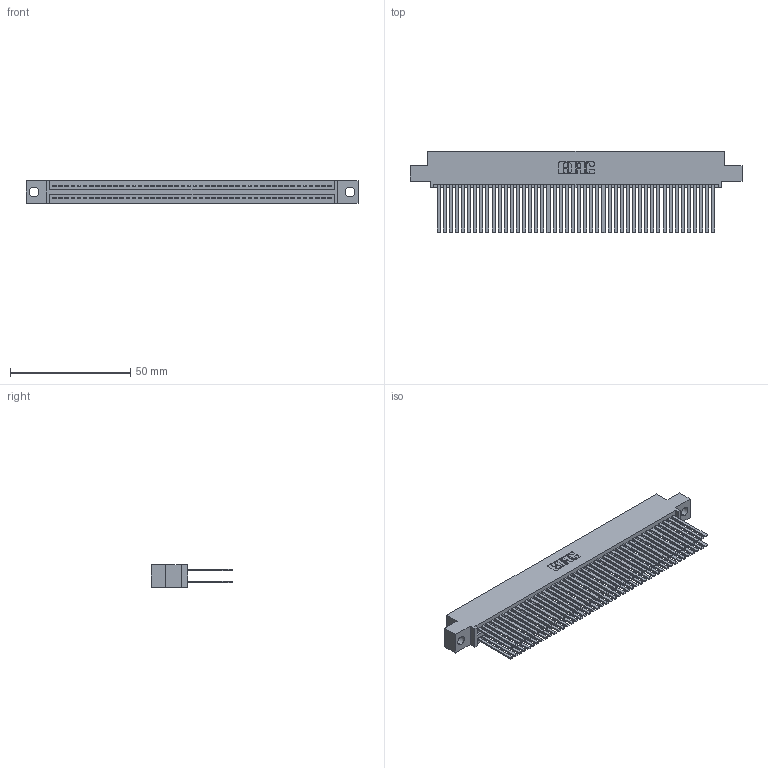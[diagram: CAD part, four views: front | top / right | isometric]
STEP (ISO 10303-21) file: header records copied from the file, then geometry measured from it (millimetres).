
FILE_DESCRIPTION (( 'STEP AP203' ), '1' );
FILE_NAME ('345-092-544-504.STEP', '2018-10-04T21:38:35', ( '' ), ( '' ), 'SwSTEP 2.0', 'SolidWorks 2016', '' );
FILE_SCHEMA (( 'CONFIG_CONTROL_DESIGN' ));
Length unit declared in the file: inch
Products named in the file (3): 345-292-001_345-293-144; 345-092-544-504; 345 Part_0.110 Offset - 0.156 Dia-TH
Assembly tree (93 placements, depth 2):
  345-092-544-504
    345 Part_0.110 Offset - 0.156 Dia-TH
    345-292-001_345-293-144  x92
Bounding box: 138.05 x 33.96 x 9.4 mm (x, y, z)
Volume: 14575.8 mm3; surface area: 25310.9 mm2
Topology: 93 solids, 93 shells, 4178 faces, 12405 edges, 8146 vertices
Faces by surface type: plane 2752, cylinder 1426
Entity records: 35505 total; most frequent: CARTESIAN_POINT 5948, ORIENTED_EDGE 5882, DIRECTION 5237, EDGE_CURVE 2941, LINE 2629, VECTOR 2629, VERTEX_POINT 1958, AXIS2_PLACEMENT_3D 1304
